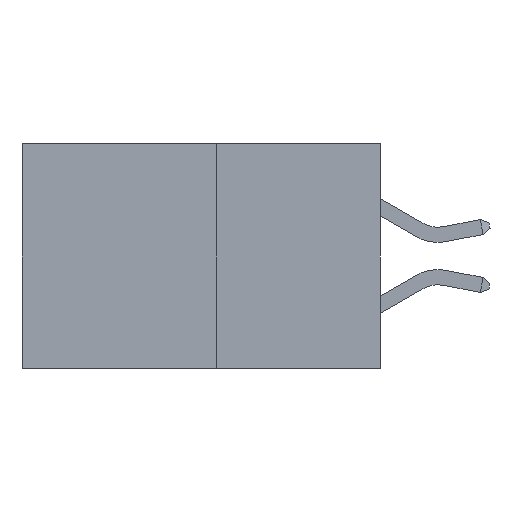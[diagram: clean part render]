
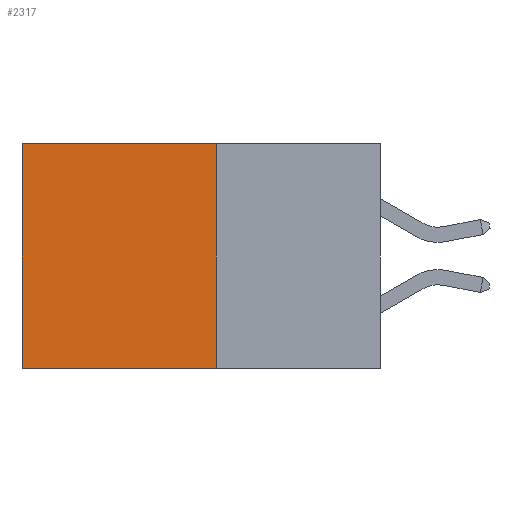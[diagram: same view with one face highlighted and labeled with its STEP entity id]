
A CAD part, left-side view. The second image highlights one B-rep face of the part: STEP entity #2317.
In plain terms, the highlighted planar face has unit normal (-1, 0, 0).
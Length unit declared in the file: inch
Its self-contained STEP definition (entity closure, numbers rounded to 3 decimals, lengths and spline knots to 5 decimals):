
#15 = CARTESIAN_POINT ( 'NONE',  ( 0.277, 0.27, 0. ) ) ;
#468 = EDGE_CURVE ( 'NONE', #16169, #10564, #1748, .T. ) ;
#1313 = CARTESIAN_POINT ( 'NONE',  ( 0.277, 0.59, -0.37 ) ) ;
#1748 = LINE ( 'NONE', #1313, #16202 ) ;
#1958 = ORIENTED_EDGE ( 'NONE', *, *, #13856, .F. ) ;
#2317 = ADVANCED_FACE ( 'NONE', ( #28589 ), #23721, .F. ) ;
#3345 = CARTESIAN_POINT ( 'NONE',  ( 0.277, 0.27, 0. ) ) ;
#4248 = EDGE_CURVE ( 'NONE', #15169, #16169, #19324, .T. ) ;
#4900 = CARTESIAN_POINT ( 'NONE',  ( 0.277, 0.27, -0.37 ) ) ;
#6095 = ORIENTED_EDGE ( 'NONE', *, *, #9932, .F. ) ;
#7851 = CARTESIAN_POINT ( 'NONE',  ( 0.277, 0.59, -0.37 ) ) ;
#8546 = ORIENTED_EDGE ( 'NONE', *, *, #468, .T. ) ;
#8825 = DIRECTION ( 'NONE',  ( 0., 1., 0. ) ) ;
#9932 = EDGE_CURVE ( 'NONE', #15169, #19657, #16896, .T. ) ;
#10564 = VERTEX_POINT ( 'NONE', #7851 ) ;
#11379 = DIRECTION ( 'NONE',  ( 0., 0., -1. ) ) ;
#12902 = LINE ( 'NONE', #30335, #26305 ) ;
#13856 = EDGE_CURVE ( 'NONE', #19657, #10564, #12902, .T. ) ;
#14466 = EDGE_LOOP ( 'NONE', ( #8546, #1958, #6095, #25800 ) ) ;
#15169 = VERTEX_POINT ( 'NONE', #3345 ) ;
#16169 = VERTEX_POINT ( 'NONE', #28797 ) ;
#16202 = VECTOR ( 'NONE', #11379, 39.37008 ) ;
#16621 = DIRECTION ( 'NONE',  ( 0., 1., 0. ) ) ;
#16896 = LINE ( 'NONE', #32220, #23126 ) ;
#18788 = DIRECTION ( 'NONE',  ( 0., 0., -1. ) ) ;
#19324 = LINE ( 'NONE', #15, #34726 ) ;
#19657 = VERTEX_POINT ( 'NONE', #4900 ) ;
#23126 = VECTOR ( 'NONE', #18788, 39.37008 ) ;
#23232 = DIRECTION ( 'NONE',  ( 0., 0., -1. ) ) ;
#23264 = DIRECTION ( 'NONE',  ( 1., 0., 0. ) ) ;
#23721 = PLANE ( 'NONE',  #29674 ) ;
#24334 = CARTESIAN_POINT ( 'NONE',  ( 0.277, 0.27, -0.37 ) ) ;
#25800 = ORIENTED_EDGE ( 'NONE', *, *, #4248, .T. ) ;
#26305 = VECTOR ( 'NONE', #8825, 39.37008 ) ;
#28589 = FACE_OUTER_BOUND ( 'NONE', #14466, .T. ) ;
#28797 = CARTESIAN_POINT ( 'NONE',  ( 0.277, 0.59, 0. ) ) ;
#29674 = AXIS2_PLACEMENT_3D ( 'NONE', #24334, #23264, #23232 ) ;
#30335 = CARTESIAN_POINT ( 'NONE',  ( 0.277, 0.27, -0.37 ) ) ;
#32220 = CARTESIAN_POINT ( 'NONE',  ( 0.277, 0.27, -0.37 ) ) ;
#34726 = VECTOR ( 'NONE', #16621, 39.37008 ) ;
